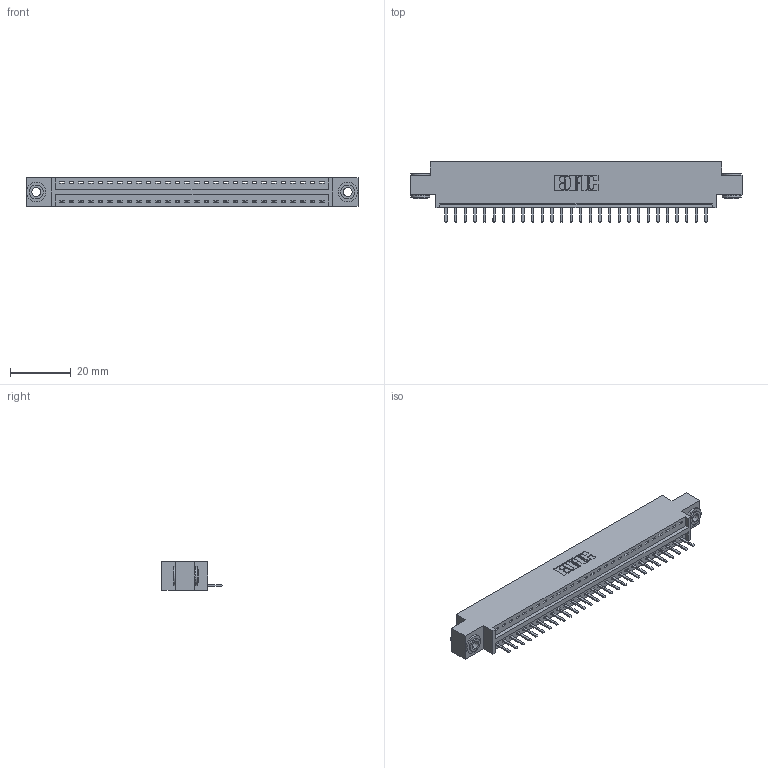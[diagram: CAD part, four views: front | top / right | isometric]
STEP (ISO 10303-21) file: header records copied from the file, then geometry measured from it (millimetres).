
FILE_DESCRIPTION (( 'STEP AP203' ), '1' );
FILE_NAME ('346-028-520-603.STEP', '2022-05-06T06:14:58', ( '' ), ( '' ), 'SwSTEP 2.0', 'SolidWorks 2020', '' );
FILE_SCHEMA (( 'CONFIG_CONTROL_DESIGN' ));
Length unit declared in the file: inch
Products named in the file (4): 345-292-001_345-293-120; 346 Part_0.170 Offset - 0.156 Dia-TH; 345-250-002_345-250-002-102; 346-028-520-603
Assembly tree (31 placements, depth 2):
  346-028-520-603
    346 Part_0.170 Offset - 0.156 Dia-TH
    345-292-001_345-293-120  x28
    345-250-002_345-250-002-102  x2
Bounding box: 109.47 x 20.02 x 9.4 mm (x, y, z)
Volume: 10148.8 mm3; surface area: 12676.5 mm2
Topology: 31 solids, 31 shells, 1914 faces, 5605 edges, 3658 vertices
Faces by surface type: plane 1280, cylinder 626, cone 8
Entity records: 20574 total; most frequent: CARTESIAN_POINT 3525, ORIENTED_EDGE 3466, DIRECTION 3143, EDGE_CURVE 1733, VECTOR 1461, LINE 1461, VERTEX_POINT 1150, AXIS2_PLACEMENT_3D 841
